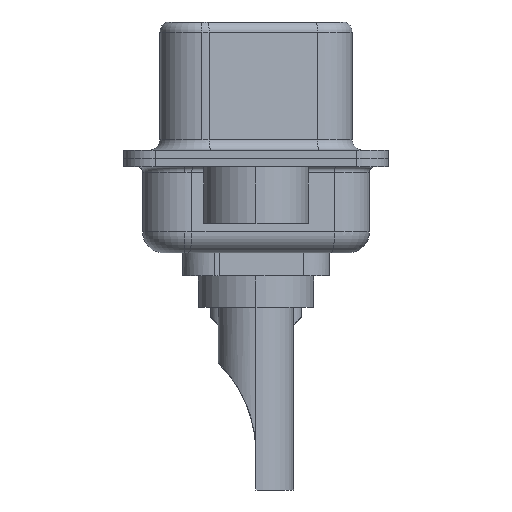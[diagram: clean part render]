
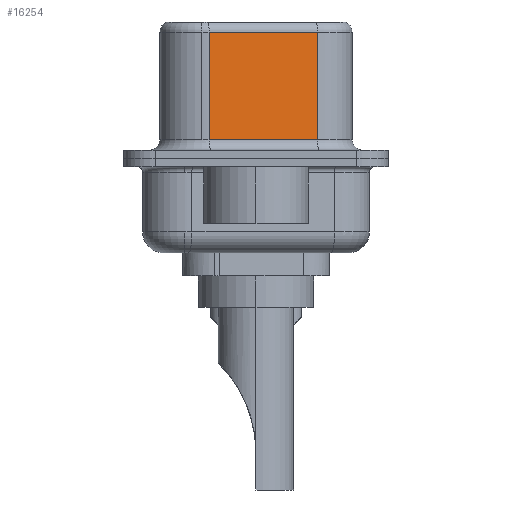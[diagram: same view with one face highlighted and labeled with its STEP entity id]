
A CAD part, left-side view. The second image highlights one B-rep face of the part: STEP entity #16254.
In plain terms, the highlighted planar face has unit normal (-0.985, -0.174, 0).
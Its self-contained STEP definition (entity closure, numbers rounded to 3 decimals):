
#862 = CARTESIAN_POINT ( 'NONE',  ( 3.655, 2.233, 6.02 ) ) ;
#1023 = DIRECTION ( 'NONE',  ( -0.174, 0.985, 0. ) ) ;
#1987 = FACE_OUTER_BOUND ( 'NONE', #14766, .T. ) ;
#2476 = CARTESIAN_POINT ( 'NONE',  ( 4.565, -2.927, 6.02 ) ) ;
#2986 = LINE ( 'NONE', #10971, #14025 ) ;
#3552 = VECTOR ( 'NONE', #1023, 1000. ) ;
#3695 = DIRECTION ( 'NONE',  ( 0.174, -0.985, 0. ) ) ;
#3869 = VECTOR ( 'NONE', #3695, 1000. ) ;
#3946 = PLANE ( 'NONE',  #14784 ) ;
#5172 = CARTESIAN_POINT ( 'NONE',  ( 4.565, -2.927, 0.9 ) ) ;
#5251 = VERTEX_POINT ( 'NONE', #15825 ) ;
#5371 = DIRECTION ( 'NONE',  ( 0.985, 0.174, 0. ) ) ;
#5740 = CARTESIAN_POINT ( 'NONE',  ( 3.655, 2.233, 0.9 ) ) ;
#7431 = CARTESIAN_POINT ( 'NONE',  ( 3.655, 2.233, 6.52 ) ) ;
#9302 = ORIENTED_EDGE ( 'NONE', *, *, #11917, .F. ) ;
#9348 = EDGE_CURVE ( 'NONE', #5251, #14398, #11191, .T. ) ;
#10347 = LINE ( 'NONE', #7431, #17554 ) ;
#10451 = ORIENTED_EDGE ( 'NONE', *, *, #11861, .T. ) ;
#10971 = CARTESIAN_POINT ( 'NONE',  ( 4.565, -2.927, 6.52 ) ) ;
#11191 = LINE ( 'NONE', #2476, #3552 ) ;
#11861 = EDGE_CURVE ( 'NONE', #13440, #11896, #14905, .T. ) ;
#11867 = DIRECTION ( 'NONE',  ( 0., 0., -1. ) ) ;
#11896 = VERTEX_POINT ( 'NONE', #5172 ) ;
#11917 = EDGE_CURVE ( 'NONE', #5251, #11896, #2986, .T. ) ;
#13440 = VERTEX_POINT ( 'NONE', #5740 ) ;
#13770 = CARTESIAN_POINT ( 'NONE',  ( 4.565, -2.927, 0.9 ) ) ;
#13830 = DIRECTION ( 'NONE',  ( 0., 0., -1. ) ) ;
#14025 = VECTOR ( 'NONE', #13830, 1000. ) ;
#14039 = CARTESIAN_POINT ( 'NONE',  ( 4.565, -2.927, 6.52 ) ) ;
#14104 = EDGE_CURVE ( 'NONE', #14398, #13440, #10347, .T. ) ;
#14398 = VERTEX_POINT ( 'NONE', #862 ) ;
#14731 = ORIENTED_EDGE ( 'NONE', *, *, #9348, .T. ) ;
#14766 = EDGE_LOOP ( 'NONE', ( #9302, #14731, #18554, #10451 ) ) ;
#14784 = AXIS2_PLACEMENT_3D ( 'NONE', #14039, #5371, #15442 ) ;
#14905 = LINE ( 'NONE', #13770, #3869 ) ;
#15442 = DIRECTION ( 'NONE',  ( -0.174, 0.985, 0. ) ) ;
#15825 = CARTESIAN_POINT ( 'NONE',  ( 4.565, -2.927, 6.02 ) ) ;
#16254 = ADVANCED_FACE ( 'NONE', ( #1987 ), #3946, .F. ) ;
#17554 = VECTOR ( 'NONE', #11867, 1000. ) ;
#18554 = ORIENTED_EDGE ( 'NONE', *, *, #14104, .T. ) ;
